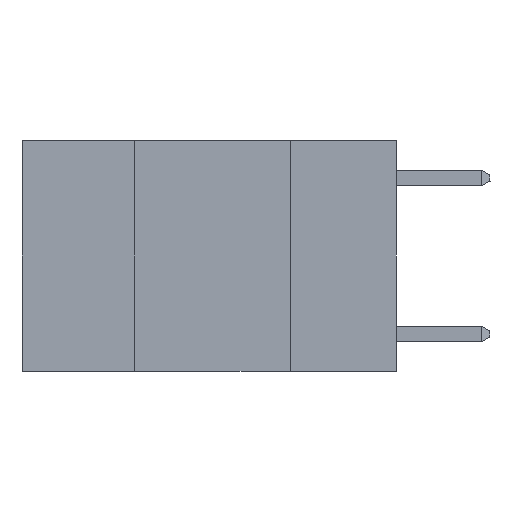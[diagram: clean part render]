
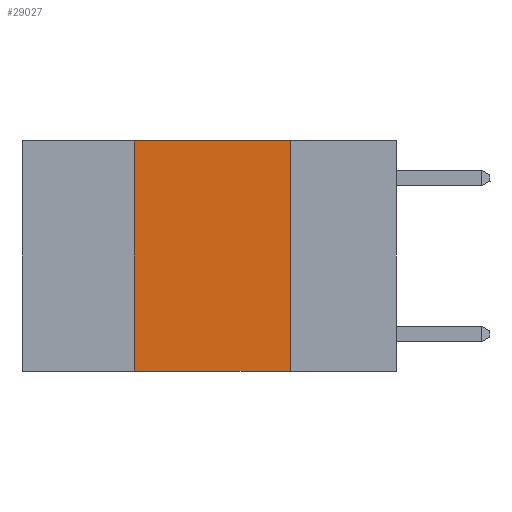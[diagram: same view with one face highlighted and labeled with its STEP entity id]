
A CAD part, left-side view. The second image highlights one B-rep face of the part: STEP entity #29027.
In plain terms, the highlighted planar face has unit normal (-1, 0, 0).
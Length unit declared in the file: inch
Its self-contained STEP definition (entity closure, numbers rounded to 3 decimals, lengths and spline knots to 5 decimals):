
#288 = VERTEX_POINT ( 'NONE', #26853 ) ;
#1770 = CARTESIAN_POINT ( 'NONE',  ( 0., 0.6, -0.37 ) ) ;
#3419 = LINE ( 'NONE', #1770, #10219 ) ;
#3569 = CARTESIAN_POINT ( 'NONE',  ( 0., 0.42, -0.37 ) ) ;
#4261 = PLANE ( 'NONE',  #27855 ) ;
#4734 = DIRECTION ( 'NONE',  ( 0., 0., 1. ) ) ;
#5406 = DIRECTION ( 'NONE',  ( 0., 0., -1. ) ) ;
#6475 = ORIENTED_EDGE ( 'NONE', *, *, #24103, .T. ) ;
#7712 = DIRECTION ( 'NONE',  ( 1., 0., 0. ) ) ;
#8701 = DIRECTION ( 'NONE',  ( 0., -1., 0. ) ) ;
#10037 = ORIENTED_EDGE ( 'NONE', *, *, #17510, .F. ) ;
#10219 = VECTOR ( 'NONE', #16956, 39.37008 ) ;
#10226 = LINE ( 'NONE', #17334, #16897 ) ;
#12420 = ORIENTED_EDGE ( 'NONE', *, *, #27431, .F. ) ;
#12439 = CARTESIAN_POINT ( 'NONE',  ( 0., 0.17, -0.37 ) ) ;
#16897 = VECTOR ( 'NONE', #4734, 39.37008 ) ;
#16956 = DIRECTION ( 'NONE',  ( 0., -1., 0. ) ) ;
#16966 = VECTOR ( 'NONE', #5406, 39.37008 ) ;
#17325 = VERTEX_POINT ( 'NONE', #12439 ) ;
#17334 = CARTESIAN_POINT ( 'NONE',  ( 0., 0.42, 0. ) ) ;
#17510 = EDGE_CURVE ( 'NONE', #288, #17325, #24288, .T. ) ;
#20489 = CARTESIAN_POINT ( 'NONE',  ( 0., 0.17, 0. ) ) ;
#21815 = VECTOR ( 'NONE', #8701, 39.37008 ) ;
#22681 = CARTESIAN_POINT ( 'NONE',  ( 0., 0.6, 0. ) ) ;
#23634 = CARTESIAN_POINT ( 'NONE',  ( 0., 0.6, 0. ) ) ;
#23921 = VERTEX_POINT ( 'NONE', #3569 ) ;
#24103 = EDGE_CURVE ( 'NONE', #23921, #17325, #3419, .T. ) ;
#24288 = LINE ( 'NONE', #20489, #16966 ) ;
#25147 = DIRECTION ( 'NONE',  ( 0., 0., -1. ) ) ;
#26249 = CARTESIAN_POINT ( 'NONE',  ( 0., 0.42, 0. ) ) ;
#26853 = CARTESIAN_POINT ( 'NONE',  ( 0., 0.17, 0. ) ) ;
#27431 = EDGE_CURVE ( 'NONE', #23921, #31471, #10226, .T. ) ;
#27601 = LINE ( 'NONE', #23634, #21815 ) ;
#27855 = AXIS2_PLACEMENT_3D ( 'NONE', #22681, #7712, #25147 ) ;
#28581 = EDGE_LOOP ( 'NONE', ( #10037, #30602, #12420, #6475 ) ) ;
#28772 = FACE_OUTER_BOUND ( 'NONE', #28581, .T. ) ;
#29027 = ADVANCED_FACE ( 'NONE', ( #28772 ), #4261, .F. ) ;
#29275 = EDGE_CURVE ( 'NONE', #31471, #288, #27601, .T. ) ;
#30602 = ORIENTED_EDGE ( 'NONE', *, *, #29275, .F. ) ;
#31471 = VERTEX_POINT ( 'NONE', #26249 ) ;
